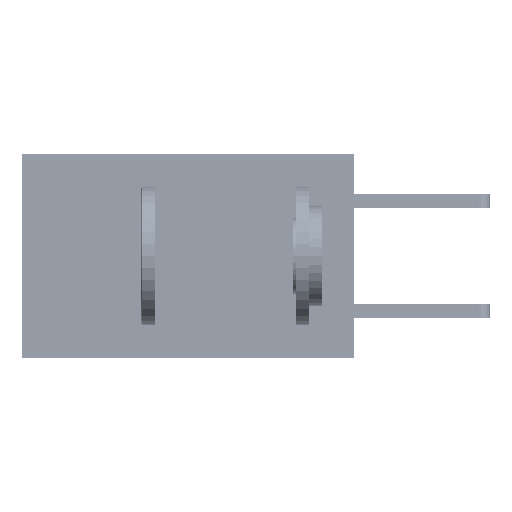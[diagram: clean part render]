
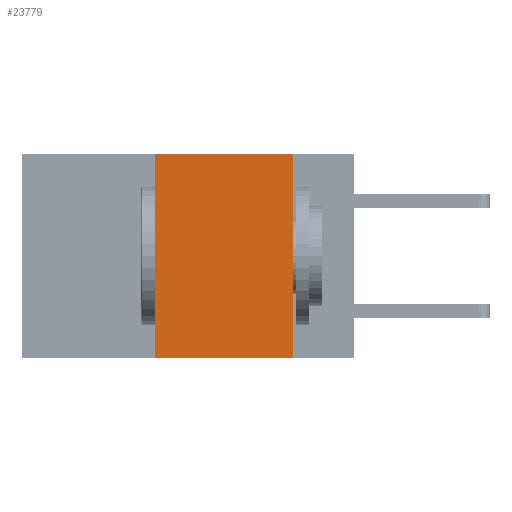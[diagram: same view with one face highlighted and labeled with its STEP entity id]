
A CAD part, left-side view. The second image highlights one B-rep face of the part: STEP entity #23779.
In plain terms, the highlighted planar face has unit normal (-1, 0, 0).
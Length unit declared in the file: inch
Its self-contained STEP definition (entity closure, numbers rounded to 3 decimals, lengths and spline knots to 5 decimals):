
#459 = VERTEX_POINT ( 'NONE', #18747 ) ;
#690 = EDGE_CURVE ( 'NONE', #12214, #37381, #32620, .T. ) ;
#1552 = ORIENTED_EDGE ( 'NONE', *, *, #5559, .F. ) ;
#3714 = LINE ( 'NONE', #45272, #32538 ) ;
#4215 = CARTESIAN_POINT ( 'NONE',  ( 0., 0.36, -0.37 ) ) ;
#4614 = CARTESIAN_POINT ( 'NONE',  ( 0., 0.6, -0.37 ) ) ;
#4877 = LINE ( 'NONE', #4614, #42151 ) ;
#5559 = EDGE_CURVE ( 'NONE', #25783, #459, #3714, .T. ) ;
#7573 = CARTESIAN_POINT ( 'NONE',  ( 0., 0.11, 0. ) ) ;
#8168 = DIRECTION ( 'NONE',  ( 0., 0., -1. ) ) ;
#10578 = DIRECTION ( 'NONE',  ( 0., -1., 0. ) ) ;
#12211 = VECTOR ( 'NONE', #8168, 39.37008 ) ;
#12214 = VERTEX_POINT ( 'NONE', #25907 ) ;
#14286 = DIRECTION ( 'NONE',  ( 1., 0., 0. ) ) ;
#18747 = CARTESIAN_POINT ( 'NONE',  ( 0., 0.36, 0. ) ) ;
#21325 = AXIS2_PLACEMENT_3D ( 'NONE', #43145, #14286, #28869 ) ;
#23779 = ADVANCED_FACE ( 'NONE', ( #37742 ), #25116, .F. ) ;
#25116 = PLANE ( 'NONE',  #21325 ) ;
#25783 = VERTEX_POINT ( 'NONE', #4215 ) ;
#25787 = DIRECTION ( 'NONE',  ( 0., 0., 1. ) ) ;
#25907 = CARTESIAN_POINT ( 'NONE',  ( 0., 0.11, 0. ) ) ;
#26463 = ORIENTED_EDGE ( 'NONE', *, *, #690, .F. ) ;
#28620 = CARTESIAN_POINT ( 'NONE',  ( 0., 0.6, 0. ) ) ;
#28869 = DIRECTION ( 'NONE',  ( 0., 0., -1. ) ) ;
#30339 = EDGE_CURVE ( 'NONE', #459, #12214, #45098, .T. ) ;
#32538 = VECTOR ( 'NONE', #25787, 39.37008 ) ;
#32620 = LINE ( 'NONE', #7573, #12211 ) ;
#32710 = EDGE_CURVE ( 'NONE', #25783, #37381, #4877, .T. ) ;
#33564 = DIRECTION ( 'NONE',  ( 0., -1., 0. ) ) ;
#34381 = CARTESIAN_POINT ( 'NONE',  ( 0., 0.11, -0.37 ) ) ;
#35650 = VECTOR ( 'NONE', #10578, 39.37008 ) ;
#37342 = ORIENTED_EDGE ( 'NONE', *, *, #30339, .F. ) ;
#37381 = VERTEX_POINT ( 'NONE', #34381 ) ;
#37742 = FACE_OUTER_BOUND ( 'NONE', #41043, .T. ) ;
#41043 = EDGE_LOOP ( 'NONE', ( #26463, #37342, #1552, #41672 ) ) ;
#41672 = ORIENTED_EDGE ( 'NONE', *, *, #32710, .T. ) ;
#42151 = VECTOR ( 'NONE', #33564, 39.37008 ) ;
#43145 = CARTESIAN_POINT ( 'NONE',  ( 0., 0.6, 0. ) ) ;
#45098 = LINE ( 'NONE', #28620, #35650 ) ;
#45272 = CARTESIAN_POINT ( 'NONE',  ( 0., 0.36, 0. ) ) ;
